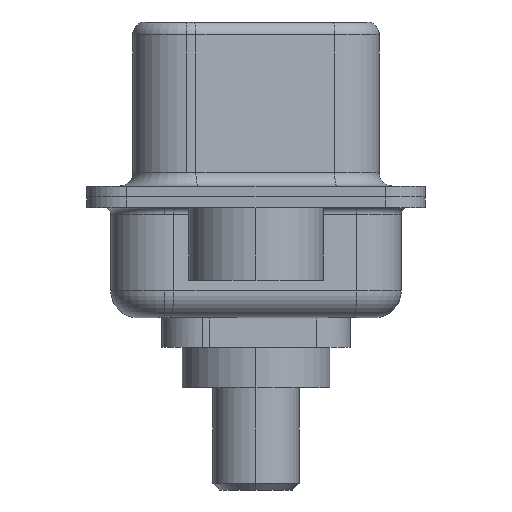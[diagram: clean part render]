
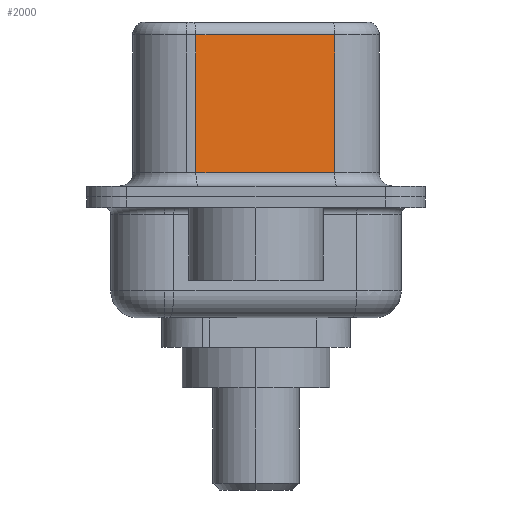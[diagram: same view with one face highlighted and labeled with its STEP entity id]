
A CAD part, left-side view. The second image highlights one B-rep face of the part: STEP entity #2000.
In plain terms, the highlighted planar face has unit normal (-0.985, -0.174, 0).
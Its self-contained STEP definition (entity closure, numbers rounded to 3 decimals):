
#186 = EDGE_CURVE ( 'NONE', #4913, #7293, #5377, .T. ) ;
#245 = ORIENTED_EDGE ( 'NONE', *, *, #9032, .T. ) ;
#256 = DIRECTION ( 'NONE',  ( -0.174, 0.985, 0. ) ) ;
#694 = VECTOR ( 'NONE', #9858, 1000. ) ;
#978 = EDGE_CURVE ( 'NONE', #4913, #11681, #5525, .T. ) ;
#1317 = LINE ( 'NONE', #9904, #694 ) ;
#2000 = ADVANCED_FACE ( 'NONE', ( #11080 ), #4428, .F. ) ;
#3284 = DIRECTION ( 'NONE',  ( -0.174, 0.985, 0. ) ) ;
#4036 = CARTESIAN_POINT ( 'NONE',  ( 4.565, -2.927, 6.02 ) ) ;
#4422 = ORIENTED_EDGE ( 'NONE', *, *, #12706, .T. ) ;
#4428 = PLANE ( 'NONE',  #9503 ) ;
#4913 = VERTEX_POINT ( 'NONE', #11188 ) ;
#5377 = LINE ( 'NONE', #7330, #7680 ) ;
#5525 = LINE ( 'NONE', #4036, #7809 ) ;
#6298 = LINE ( 'NONE', #10624, #11286 ) ;
#7188 = CARTESIAN_POINT ( 'NONE',  ( 3.655, 2.233, 6.02 ) ) ;
#7293 = VERTEX_POINT ( 'NONE', #10558 ) ;
#7330 = CARTESIAN_POINT ( 'NONE',  ( 4.565, -2.927, 6.52 ) ) ;
#7680 = VECTOR ( 'NONE', #10353, 1000. ) ;
#7809 = VECTOR ( 'NONE', #3284, 1000. ) ;
#8901 = CARTESIAN_POINT ( 'NONE',  ( 4.565, -2.927, 6.52 ) ) ;
#9032 = EDGE_CURVE ( 'NONE', #11681, #10166, #1317, .T. ) ;
#9111 = CARTESIAN_POINT ( 'NONE',  ( 3.655, 2.233, 0.9 ) ) ;
#9273 = DIRECTION ( 'NONE',  ( 0.985, 0.174, 0. ) ) ;
#9503 = AXIS2_PLACEMENT_3D ( 'NONE', #8901, #9273, #256 ) ;
#9858 = DIRECTION ( 'NONE',  ( 0., 0., -1. ) ) ;
#9904 = CARTESIAN_POINT ( 'NONE',  ( 3.655, 2.233, 6.52 ) ) ;
#10166 = VERTEX_POINT ( 'NONE', #9111 ) ;
#10353 = DIRECTION ( 'NONE',  ( 0., 0., -1. ) ) ;
#10558 = CARTESIAN_POINT ( 'NONE',  ( 4.565, -2.927, 0.9 ) ) ;
#10624 = CARTESIAN_POINT ( 'NONE',  ( 4.565, -2.927, 0.9 ) ) ;
#11080 = FACE_OUTER_BOUND ( 'NONE', #11170, .T. ) ;
#11170 = EDGE_LOOP ( 'NONE', ( #12312, #12681, #245, #4422 ) ) ;
#11188 = CARTESIAN_POINT ( 'NONE',  ( 4.565, -2.927, 6.02 ) ) ;
#11286 = VECTOR ( 'NONE', #11622, 1000. ) ;
#11622 = DIRECTION ( 'NONE',  ( 0.174, -0.985, 0. ) ) ;
#11681 = VERTEX_POINT ( 'NONE', #7188 ) ;
#12312 = ORIENTED_EDGE ( 'NONE', *, *, #186, .F. ) ;
#12681 = ORIENTED_EDGE ( 'NONE', *, *, #978, .T. ) ;
#12706 = EDGE_CURVE ( 'NONE', #10166, #7293, #6298, .T. ) ;
